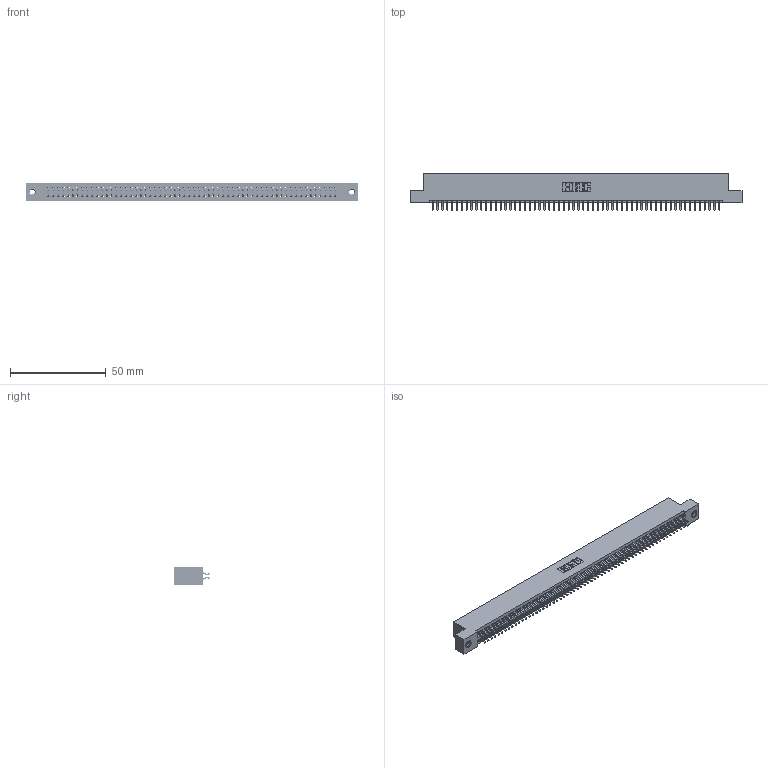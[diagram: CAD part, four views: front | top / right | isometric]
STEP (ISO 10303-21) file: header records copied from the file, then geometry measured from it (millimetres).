
FILE_DESCRIPTION (( 'STEP AP203' ), '1' );
FILE_NAME ('345-120-556-207.STEP', '2019-11-06T03:31:23', ( '' ), ( '' ), 'SwSTEP 2.0', 'SolidWorks 2016', '' );
FILE_SCHEMA (( 'CONFIG_CONTROL_DESIGN' ));
Length unit declared in the file: inch
Products named in the file (4): 345 Part_Flush Mounting Lugs - 0.156 Dia-TI; 345-250-001_345-250-005-103; 345-120-556-207; 345-292-001_556 Tail
Assembly tree (123 placements, depth 2):
  345-120-556-207
    345 Part_Flush Mounting Lugs - 0.156 Dia-TI
    345-292-001_556 Tail  x120
    345-250-001_345-250-005-103  x2
Bounding box: 173.61 x 19.24 x 9.4 mm (x, y, z)
Volume: 17013.4 mm3; surface area: 25420.1 mm2
Topology: 123 solids, 123 shells, 6906 faces, 20517 edges, 13510 vertices
Faces by surface type: plane 4552, cylinder 2338, cone 12, torus 4
Entity records: 46060 total; most frequent: CARTESIAN_POINT 7699, ORIENTED_EDGE 7614, DIRECTION 6781, EDGE_CURVE 3807, VECTOR 3407, LINE 3407, VERTEX_POINT 2532, AXIS2_PLACEMENT_3D 1687
